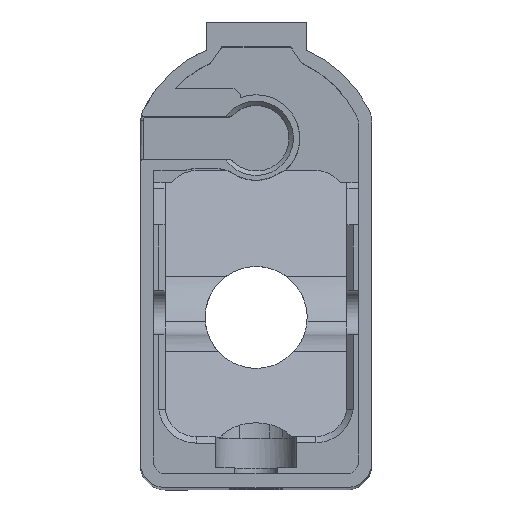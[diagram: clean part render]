
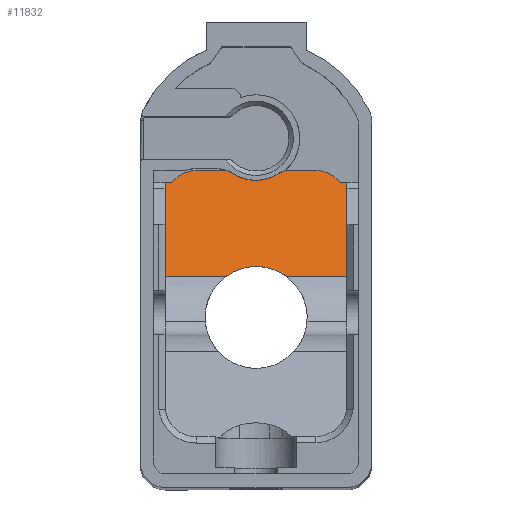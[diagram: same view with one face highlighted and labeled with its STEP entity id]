
A CAD part, top view. The second image highlights one B-rep face of the part: STEP entity #11832.
In plain terms, the highlighted planar face has unit normal (0, 0.832, 0.555).
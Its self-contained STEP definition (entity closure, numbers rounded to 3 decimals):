
#978=ELLIPSE('',#12573,9.014,5.);
#979=ELLIPSE('',#12577,9.014,5.);
#984=ELLIPSE('',#12788,14.693,8.15);
#1547=FACE_OUTER_BOUND('',#2204,.T.);
#2204=EDGE_LOOP('',(#10539,#10540,#10541,#10542,#10543,#10544,#10545,#10546,
#10547,#10548,#10549,#10550,#10551,#10552,#10553,#10554,#10555,#10556));
#2309=LINE('',#16063,#3450);
#2472=LINE('',#16717,#3613);
#2538=LINE('',#16940,#3679);
#2544=LINE('',#16966,#3685);
#2821=LINE('',#18422,#3962);
#2826=LINE('',#18433,#3967);
#2933=LINE('',#18980,#4074);
#2939=LINE('',#19047,#4080);
#3034=LINE('',#19599,#4175);
#3050=LINE('',#19643,#4191);
#3117=LINE('',#20901,#4258);
#3328=LINE('',#21563,#4469);
#3329=LINE('',#21579,#4470);
#3330=LINE('',#21582,#4471);
#3331=LINE('',#21583,#4472);
#3450=VECTOR('',#12957,10.);
#3613=VECTOR('',#13320,10.);
#3679=VECTOR('',#13508,10.);
#3685=VECTOR('',#13520,10.);
#3962=VECTOR('',#14287,10.);
#3967=VECTOR('',#14298,10.);
#4074=VECTOR('',#14605,10.);
#4080=VECTOR('',#14619,10.);
#4175=VECTOR('',#14842,10.);
#4191=VECTOR('',#14876,10.);
#4258=VECTOR('',#15071,10.);
#4469=VECTOR('',#15700,10.);
#4470=VECTOR('',#15707,10.);
#4471=VECTOR('',#15712,10.);
#4472=VECTOR('',#15713,10.);
#4608=VERTEX_POINT('',#16060);
#4609=VERTEX_POINT('',#16062);
#4800=VERTEX_POINT('',#16715);
#4801=VERTEX_POINT('',#16716);
#4877=VERTEX_POINT('',#16937);
#4884=VERTEX_POINT('',#16962);
#4886=VERTEX_POINT('',#16965);
#5189=VERTEX_POINT('',#18419);
#5272=VERTEX_POINT('',#18976);
#5273=VERTEX_POINT('',#18978);
#5361=VERTEX_POINT('',#19598);
#5372=VERTEX_POINT('',#19642);
#5472=VERTEX_POINT('',#20865);
#5473=VERTEX_POINT('',#20884);
#5619=VERTEX_POINT('',#21553);
#5620=VERTEX_POINT('',#21562);
#5621=VERTEX_POINT('',#21566);
#5622=VERTEX_POINT('',#21577);
#5738=EDGE_CURVE('',#4608,#4609,#2309,.T.);
#5968=EDGE_CURVE('',#4800,#4801,#2472,.T.);
#6073=EDGE_CURVE('',#4608,#4877,#2538,.T.);
#6082=EDGE_CURVE('',#4884,#4886,#2544,.T.);
#6528=EDGE_CURVE('',#5189,#4801,#2821,.T.);
#6534=EDGE_CURVE('',#5189,#4884,#2826,.T.);
#6696=EDGE_CURVE('',#5273,#5272,#2933,.T.);
#6707=EDGE_CURVE('',#5272,#4877,#2939,.T.);
#6850=EDGE_CURVE('',#5361,#4800,#3034,.T.);
#6870=EDGE_CURVE('',#4609,#5372,#3050,.T.);
#7034=EDGE_CURVE('',#5472,#5361,#978,.T.);
#7036=EDGE_CURVE('',#5473,#5472,#3117,.T.);
#7040=EDGE_CURVE('',#5372,#5473,#979,.T.);
#7333=EDGE_CURVE('',#5619,#5620,#3328,.T.);
#7337=EDGE_CURVE('',#5622,#5621,#3329,.T.);
#7338=EDGE_CURVE('',#5619,#5621,#984,.T.);
#7339=EDGE_CURVE('',#4886,#5622,#3330,.T.);
#7340=EDGE_CURVE('',#5620,#5273,#3331,.T.);
#10539=ORIENTED_EDGE('',*,*,#7338,.T.);
#10540=ORIENTED_EDGE('',*,*,#7337,.F.);
#10541=ORIENTED_EDGE('',*,*,#7339,.F.);
#10542=ORIENTED_EDGE('',*,*,#6082,.F.);
#10543=ORIENTED_EDGE('',*,*,#6534,.F.);
#10544=ORIENTED_EDGE('',*,*,#6528,.T.);
#10545=ORIENTED_EDGE('',*,*,#5968,.F.);
#10546=ORIENTED_EDGE('',*,*,#6850,.F.);
#10547=ORIENTED_EDGE('',*,*,#7034,.F.);
#10548=ORIENTED_EDGE('',*,*,#7036,.F.);
#10549=ORIENTED_EDGE('',*,*,#7040,.F.);
#10550=ORIENTED_EDGE('',*,*,#6870,.F.);
#10551=ORIENTED_EDGE('',*,*,#5738,.F.);
#10552=ORIENTED_EDGE('',*,*,#6073,.T.);
#10553=ORIENTED_EDGE('',*,*,#6707,.F.);
#10554=ORIENTED_EDGE('',*,*,#6696,.F.);
#10555=ORIENTED_EDGE('',*,*,#7340,.F.);
#10556=ORIENTED_EDGE('',*,*,#7333,.F.);
#11237=PLANE('',#12787);
#11832=ADVANCED_FACE('',(#1547),#11237,.F.);
#12573=AXIS2_PLACEMENT_3D('',#20882,#15067,#15068);
#12577=AXIS2_PLACEMENT_3D('',#20917,#15078,#15079);
#12787=AXIS2_PLACEMENT_3D('',#21580,#15708,#15709);
#12788=AXIS2_PLACEMENT_3D('',#21581,#15710,#15711);
#12957=DIRECTION('',(0.,-0.555,0.832));
#13320=DIRECTION('',(-0.021,-0.555,0.832));
#13508=DIRECTION('',(-1.,0.,0.));
#13520=DIRECTION('',(-1.,0.,0.));
#14287=DIRECTION('',(-1.,0.,0.));
#14298=DIRECTION('',(0.,-0.555,0.832));
#14605=DIRECTION('',(-1.,0.,0.));
#14619=DIRECTION('',(0.,0.555,-0.832));
#14842=DIRECTION('',(0.,-0.555,0.832));
#14876=DIRECTION('',(0.,0.555,-0.832));
#15067=DIRECTION('center_axis',(0.,-0.832,
-0.555));
#15068=DIRECTION('ref_axis',(0.,0.555,-0.832));
#15071=DIRECTION('',(1.,0.006,-0.009));
#15078=DIRECTION('center_axis',(0.,-0.832,
-0.555));
#15079=DIRECTION('ref_axis',(0.,-0.555,0.832));
#15700=DIRECTION('',(-1.,0.,0.));
#15707=DIRECTION('',(-1.,0.,0.));
#15708=DIRECTION('center_axis',(0.,-0.832,
-0.555));
#15709=DIRECTION('ref_axis',(0.,-0.555,0.832));
#15710=DIRECTION('center_axis',(0.,-0.832,
-0.555));
#15711=DIRECTION('ref_axis',(0.,0.555,-0.832));
#15712=DIRECTION('',(0.,-0.555,0.832));
#15713=DIRECTION('',(0.,0.555,-0.832));
#16060=CARTESIAN_POINT('',(4.135,37.92,-116.942));
#16062=CARTESIAN_POINT('',(4.136,36.524,-114.849));
#16063=CARTESIAN_POINT('',(4.136,19.629,-89.506));
#16715=CARTESIAN_POINT('',(33.22,37.989,-117.046));
#16716=CARTESIAN_POINT('',(33.217,37.92,-116.942));
#16717=CARTESIAN_POINT('',(32.722,24.634,-97.013));
#16937=CARTESIAN_POINT('',(0.836,37.92,-116.942));
#16940=CARTESIAN_POINT('',(37.22,37.92,-116.942));
#16962=CARTESIAN_POINT('',(36.52,27.92,-101.942));
#16965=CARTESIAN_POINT('',(33.22,27.92,-101.942));
#16966=CARTESIAN_POINT('',(37.22,27.92,-101.942));
#18419=CARTESIAN_POINT('',(36.52,37.92,-116.942));
#18422=CARTESIAN_POINT('',(37.22,37.92,-116.942));
#18433=CARTESIAN_POINT('',(36.52,14.308,-81.524));
#18976=CARTESIAN_POINT('',(0.836,27.92,-101.942));
#18978=CARTESIAN_POINT('',(4.136,27.92,-101.942));
#18980=CARTESIAN_POINT('',(37.22,27.92,-101.942));
#19047=CARTESIAN_POINT('',(0.836,5.978,-69.029));
#19598=CARTESIAN_POINT('',(33.22,45.502,-128.316));
#19599=CARTESIAN_POINT('',(33.22,25.02,-97.593));
#19642=CARTESIAN_POINT('',(4.136,45.461,-128.254));
#19643=CARTESIAN_POINT('',(4.136,37.92,-116.942));
#20865=CARTESIAN_POINT('',(33.03,46.866,-130.361));
#20882=CARTESIAN_POINT('Origin',(28.22,45.502,-128.316));
#20884=CARTESIAN_POINT('',(4.309,46.702,-130.116));
#20901=CARTESIAN_POINT('',(32.217,46.861,-130.354));
#20917=CARTESIAN_POINT('Origin',(9.135,45.394,-128.153));
#21553=CARTESIAN_POINT('',(13.852,23.963,-96.006));
#21562=CARTESIAN_POINT('',(4.136,23.963,-96.006));
#21563=CARTESIAN_POINT('',(37.22,23.963,-96.006));
#21566=CARTESIAN_POINT('',(23.552,23.963,-96.006));
#21577=CARTESIAN_POINT('',(33.22,23.963,-96.006));
#21579=CARTESIAN_POINT('',(37.22,23.963,-96.006));
#21580=CARTESIAN_POINT('Origin',(37.22,37.92,-116.942));
#21581=CARTESIAN_POINT('Origin',(18.702,17.413,-86.181));
#21582=CARTESIAN_POINT('',(33.22,18.41,-87.678));
#21583=CARTESIAN_POINT('',(4.136,23.641,-95.524));
